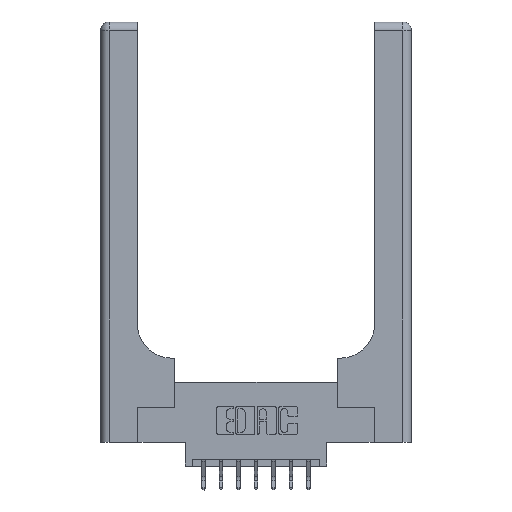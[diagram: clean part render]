
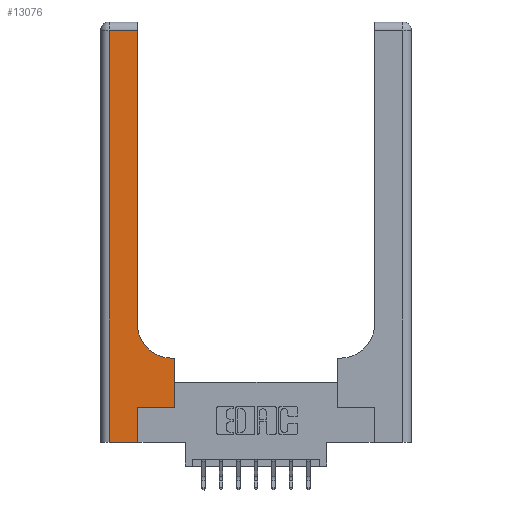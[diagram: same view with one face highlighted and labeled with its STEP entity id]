
A CAD part, top view. The second image highlights one B-rep face of the part: STEP entity #13076.
In plain terms, the highlighted planar face has unit normal (0, 0, 1).
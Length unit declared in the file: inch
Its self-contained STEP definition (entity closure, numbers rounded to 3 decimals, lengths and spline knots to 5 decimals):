
#162 = VERTEX_POINT ( 'NONE', #7956 ) ;
#343 = EDGE_CURVE ( 'NONE', #14683, #2191, #11278, .T. ) ;
#452 = CARTESIAN_POINT ( 'NONE',  ( 0., 2.94, 0.37 ) ) ;
#504 = DIRECTION ( 'NONE',  ( -1., 0., 0. ) ) ;
#620 = LINE ( 'NONE', #12481, #9070 ) ;
#918 = CARTESIAN_POINT ( 'NONE',  ( 0.528, 0.25, 0.37 ) ) ;
#995 = CIRCLE ( 'NONE', #14792, 0.25 ) ;
#1023 = EDGE_CURVE ( 'NONE', #3845, #14683, #14688, .T. ) ;
#1053 = VECTOR ( 'NONE', #12218, 39.37008 ) ;
#1171 = LINE ( 'NONE', #9413, #7263 ) ;
#1310 = LINE ( 'NONE', #7064, #13495 ) ;
#1563 = ORIENTED_EDGE ( 'NONE', *, *, #1023, .T. ) ;
#1980 = LINE ( 'NONE', #14495, #13799 ) ;
#2191 = VERTEX_POINT ( 'NONE', #13715 ) ;
#2485 = FACE_OUTER_BOUND ( 'NONE', #13581, .T. ) ;
#2517 = VECTOR ( 'NONE', #504, 39.37008 ) ;
#2916 = ORIENTED_EDGE ( 'NONE', *, *, #14244, .T. ) ;
#3165 = ORIENTED_EDGE ( 'NONE', *, *, #3708, .T. ) ;
#3708 = EDGE_CURVE ( 'NONE', #4439, #162, #995, .T. ) ;
#3709 = DIRECTION ( 'NONE',  ( -1., 0., 0. ) ) ;
#3756 = LINE ( 'NONE', #5376, #1053 ) ;
#3762 = EDGE_CURVE ( 'NONE', #14285, #14344, #620, .T. ) ;
#3845 = VERTEX_POINT ( 'NONE', #10332 ) ;
#3919 = ORIENTED_EDGE ( 'NONE', *, *, #12714, .T. ) ;
#4236 = ORIENTED_EDGE ( 'NONE', *, *, #3762, .T. ) ;
#4372 = DIRECTION ( 'NONE',  ( 0., 0., -1. ) ) ;
#4439 = VERTEX_POINT ( 'NONE', #14663 ) ;
#4565 = CARTESIAN_POINT ( 'NONE',  ( 0.06, 2.94, 0.37 ) ) ;
#4701 = EDGE_CURVE ( 'NONE', #5272, #4439, #1171, .T. ) ;
#4985 = DIRECTION ( 'NONE',  ( 0., 1., 0. ) ) ;
#5190 = VECTOR ( 'NONE', #10506, 39.37008 ) ;
#5252 = ORIENTED_EDGE ( 'NONE', *, *, #343, .T. ) ;
#5272 = VERTEX_POINT ( 'NONE', #10407 ) ;
#5376 = CARTESIAN_POINT ( 'NONE',  ( 0.26, 3., 0.37 ) ) ;
#5639 = DIRECTION ( 'NONE',  ( 0., 1., 0. ) ) ;
#5933 = EDGE_CURVE ( 'NONE', #14344, #12457, #1310, .T. ) ;
#6532 = AXIS2_PLACEMENT_3D ( 'NONE', #7111, #10580, #3709 ) ;
#7064 = CARTESIAN_POINT ( 'NONE',  ( 0.265, 0.25, 0.37 ) ) ;
#7111 = CARTESIAN_POINT ( 'NONE',  ( 0., 3., 0.37 ) ) ;
#7263 = VECTOR ( 'NONE', #12858, 39.37008 ) ;
#7892 = EDGE_CURVE ( 'NONE', #2191, #14285, #1980, .T. ) ;
#7956 = CARTESIAN_POINT ( 'NONE',  ( 0.26, 0.85, 0.37 ) ) ;
#8213 = CARTESIAN_POINT ( 'NONE',  ( 0.06, 3., 0.37 ) ) ;
#8244 = DIRECTION ( 'NONE',  ( 1., 0., 0. ) ) ;
#8715 = LINE ( 'NONE', #11838, #14427 ) ;
#8803 = ORIENTED_EDGE ( 'NONE', *, *, #7892, .T. ) ;
#9070 = VECTOR ( 'NONE', #5639, 39.37008 ) ;
#9413 = CARTESIAN_POINT ( 'NONE',  ( 0.26, 0.6, 0.37 ) ) ;
#9580 = CARTESIAN_POINT ( 'NONE',  ( 0.265, 0., 0.37 ) ) ;
#9934 = DIRECTION ( 'NONE',  ( 1., 0., 0. ) ) ;
#10304 = ORIENTED_EDGE ( 'NONE', *, *, #5933, .T. ) ;
#10332 = CARTESIAN_POINT ( 'NONE',  ( 0.26, 2.94, 0.37 ) ) ;
#10407 = CARTESIAN_POINT ( 'NONE',  ( 0.528, 0.6, 0.37 ) ) ;
#10506 = DIRECTION ( 'NONE',  ( 0., -1., 0. ) ) ;
#10580 = DIRECTION ( 'NONE',  ( 0., 0., -1. ) ) ;
#11243 = CARTESIAN_POINT ( 'NONE',  ( 0.51, 0.85, 0.37 ) ) ;
#11278 = LINE ( 'NONE', #8213, #5190 ) ;
#11838 = CARTESIAN_POINT ( 'NONE',  ( 0.528, 0.25, 0.37 ) ) ;
#12030 = CARTESIAN_POINT ( 'NONE',  ( 0.265, 0.25, 0.37 ) ) ;
#12218 = DIRECTION ( 'NONE',  ( 0., 1., 0. ) ) ;
#12378 = DIRECTION ( 'NONE',  ( 1., 0., 0. ) ) ;
#12457 = VERTEX_POINT ( 'NONE', #918 ) ;
#12481 = CARTESIAN_POINT ( 'NONE',  ( 0.265, 0., 0.37 ) ) ;
#12714 = EDGE_CURVE ( 'NONE', #162, #3845, #3756, .T. ) ;
#12858 = DIRECTION ( 'NONE',  ( -1., 0., 0. ) ) ;
#13076 = ADVANCED_FACE ( 'NONE', ( #2485 ), #13957, .F. ) ;
#13420 = ORIENTED_EDGE ( 'NONE', *, *, #4701, .T. ) ;
#13495 = VECTOR ( 'NONE', #8244, 39.37008 ) ;
#13581 = EDGE_LOOP ( 'NONE', ( #3919, #1563, #5252, #8803, #4236, #10304, #2916, #13420, #3165 ) ) ;
#13715 = CARTESIAN_POINT ( 'NONE',  ( 0.06, 0., 0.37 ) ) ;
#13799 = VECTOR ( 'NONE', #9934, 39.37008 ) ;
#13957 = PLANE ( 'NONE',  #6532 ) ;
#14244 = EDGE_CURVE ( 'NONE', #12457, #5272, #8715, .T. ) ;
#14285 = VERTEX_POINT ( 'NONE', #9580 ) ;
#14344 = VERTEX_POINT ( 'NONE', #12030 ) ;
#14427 = VECTOR ( 'NONE', #4985, 39.37008 ) ;
#14495 = CARTESIAN_POINT ( 'NONE',  ( 0., 0., 0.37 ) ) ;
#14663 = CARTESIAN_POINT ( 'NONE',  ( 0.51, 0.6, 0.37 ) ) ;
#14683 = VERTEX_POINT ( 'NONE', #4565 ) ;
#14688 = LINE ( 'NONE', #452, #2517 ) ;
#14792 = AXIS2_PLACEMENT_3D ( 'NONE', #11243, #4372, #12378 ) ;
